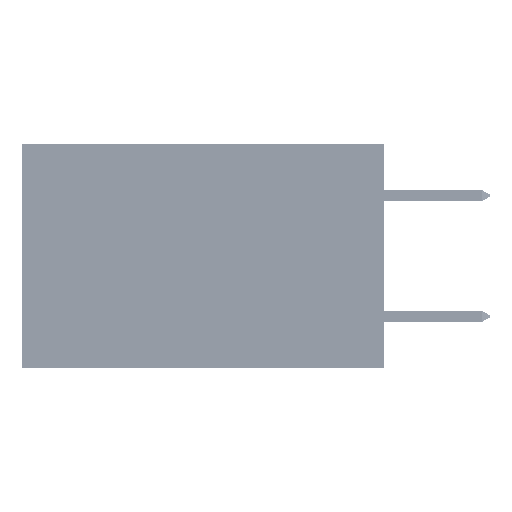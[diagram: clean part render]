
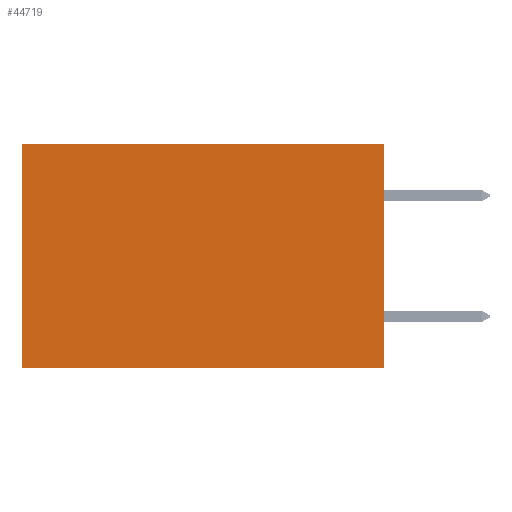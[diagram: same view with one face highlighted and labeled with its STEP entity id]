
A CAD part, left-side view. The second image highlights one B-rep face of the part: STEP entity #44719.
In plain terms, the highlighted planar face has unit normal (-1, 0, 0).
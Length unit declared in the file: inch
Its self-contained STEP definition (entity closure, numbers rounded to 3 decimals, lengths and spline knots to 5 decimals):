
#5851 = CARTESIAN_POINT ( 'NONE',  ( 0.2875, 0.6, 0. ) ) ;
#8748 = VECTOR ( 'NONE', #14949, 39.37008 ) ;
#9264 = EDGE_LOOP ( 'NONE', ( #21230, #45370, #47390, #33442 ) ) ;
#9735 = DIRECTION ( 'NONE',  ( 0., 1., 0. ) ) ;
#9983 = VERTEX_POINT ( 'NONE', #12399 ) ;
#11112 = FACE_OUTER_BOUND ( 'NONE', #9264, .T. ) ;
#11623 = LINE ( 'NONE', #36390, #8748 ) ;
#12399 = CARTESIAN_POINT ( 'NONE',  ( 0.2875, 0., -0.37 ) ) ;
#12893 = DIRECTION ( 'NONE',  ( 1., 0., 0. ) ) ;
#13728 = EDGE_CURVE ( 'NONE', #15453, #9983, #11623, .T. ) ;
#13771 = VECTOR ( 'NONE', #9735, 39.37008 ) ;
#14949 = DIRECTION ( 'NONE',  ( 0., 0., -1. ) ) ;
#15453 = VERTEX_POINT ( 'NONE', #19678 ) ;
#15634 = LINE ( 'NONE', #24443, #40999 ) ;
#15799 = PLANE ( 'NONE',  #33775 ) ;
#15957 = EDGE_CURVE ( 'NONE', #21882, #41844, #32154, .T. ) ;
#16428 = DIRECTION ( 'NONE',  ( 0., 0., -1. ) ) ;
#19678 = CARTESIAN_POINT ( 'NONE',  ( 0.2875, 0., 0. ) ) ;
#20362 = CARTESIAN_POINT ( 'NONE',  ( 0.2875, 0., -0.37 ) ) ;
#21230 = ORIENTED_EDGE ( 'NONE', *, *, #15957, .T. ) ;
#21882 = VERTEX_POINT ( 'NONE', #5851 ) ;
#24443 = CARTESIAN_POINT ( 'NONE',  ( 0.2875, 0., 0. ) ) ;
#28661 = EDGE_CURVE ( 'NONE', #15453, #21882, #15634, .T. ) ;
#29256 = VECTOR ( 'NONE', #33945, 39.37008 ) ;
#30220 = CARTESIAN_POINT ( 'NONE',  ( 0.2875, 0.6, 0. ) ) ;
#32154 = LINE ( 'NONE', #30220, #29256 ) ;
#33442 = ORIENTED_EDGE ( 'NONE', *, *, #28661, .T. ) ;
#33512 = CARTESIAN_POINT ( 'NONE',  ( 0.2875, 0.6, -0.37 ) ) ;
#33775 = AXIS2_PLACEMENT_3D ( 'NONE', #37586, #12893, #16428 ) ;
#33945 = DIRECTION ( 'NONE',  ( 0., 0., -1. ) ) ;
#36390 = CARTESIAN_POINT ( 'NONE',  ( 0.2875, 0., 0. ) ) ;
#37586 = CARTESIAN_POINT ( 'NONE',  ( 0.2875, 0., 0. ) ) ;
#39744 = LINE ( 'NONE', #20362, #13771 ) ;
#40999 = VECTOR ( 'NONE', #42831, 39.37008 ) ;
#41844 = VERTEX_POINT ( 'NONE', #33512 ) ;
#42831 = DIRECTION ( 'NONE',  ( 0., 1., 0. ) ) ;
#44719 = ADVANCED_FACE ( 'NONE', ( #11112 ), #15799, .F. ) ;
#45370 = ORIENTED_EDGE ( 'NONE', *, *, #46703, .F. ) ;
#46703 = EDGE_CURVE ( 'NONE', #9983, #41844, #39744, .T. ) ;
#47390 = ORIENTED_EDGE ( 'NONE', *, *, #13728, .F. ) ;
